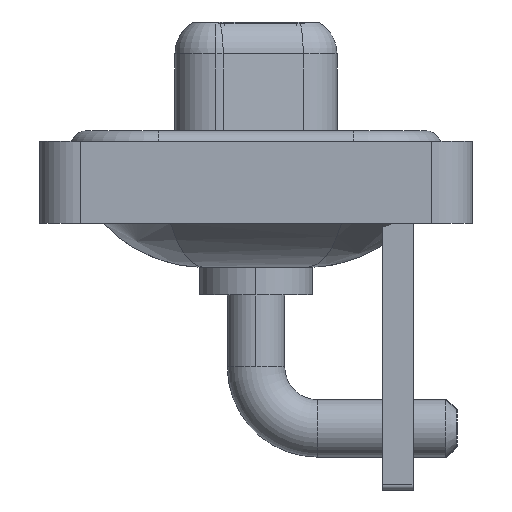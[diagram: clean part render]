
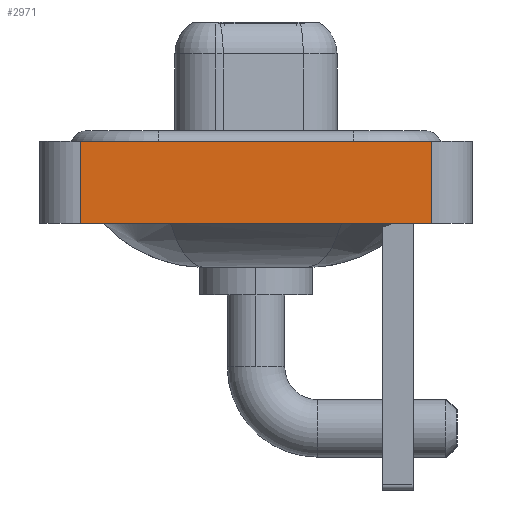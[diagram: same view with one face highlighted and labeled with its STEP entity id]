
A CAD part, left-side view. The second image highlights one B-rep face of the part: STEP entity #2971.
In plain terms, the highlighted planar face has unit normal (-1, 0, 0).
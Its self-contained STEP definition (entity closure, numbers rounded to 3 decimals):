
#791 = ORIENTED_EDGE ( 'NONE', *, *, #10012, .T. ) ;
#990 = CARTESIAN_POINT ( 'NONE',  ( -7.3, 8.55, -3.6 ) ) ;
#1152 = DIRECTION ( 'NONE',  ( 0., -1., 0. ) ) ;
#2971 = ADVANCED_FACE ( 'NONE', ( #12837 ), #17262, .T. ) ;
#3034 = CARTESIAN_POINT ( 'NONE',  ( -7.3, -8.55, -3.6 ) ) ;
#3097 = EDGE_CURVE ( 'NONE', #4671, #17338, #14737, .T. ) ;
#3956 = VECTOR ( 'NONE', #1152, 1000. ) ;
#4031 = LINE ( 'NONE', #13815, #3956 ) ;
#4326 = CARTESIAN_POINT ( 'NONE',  ( -7.3, -8.55, -3.6 ) ) ;
#4671 = VERTEX_POINT ( 'NONE', #17143 ) ;
#5493 = VERTEX_POINT ( 'NONE', #13110 ) ;
#5667 = VECTOR ( 'NONE', #5874, 1000. ) ;
#5874 = DIRECTION ( 'NONE',  ( 0., 0., 1. ) ) ;
#5879 = DIRECTION ( 'NONE',  ( 0., 0., 1. ) ) ;
#6890 = LINE ( 'NONE', #4326, #5667 ) ;
#7021 = CARTESIAN_POINT ( 'NONE',  ( -7.3, -8.55, -3.6 ) ) ;
#7369 = ORIENTED_EDGE ( 'NONE', *, *, #3097, .T. ) ;
#9213 = VECTOR ( 'NONE', #12275, 1000. ) ;
#9560 = CARTESIAN_POINT ( 'NONE',  ( -7.3, -8.55, 0.4 ) ) ;
#10012 = EDGE_CURVE ( 'NONE', #17338, #14503, #6890, .T. ) ;
#10489 = EDGE_LOOP ( 'NONE', ( #791, #13140, #17829, #7369 ) ) ;
#10796 = LINE ( 'NONE', #990, #9213 ) ;
#12275 = DIRECTION ( 'NONE',  ( 0., 0., 1. ) ) ;
#12837 = FACE_OUTER_BOUND ( 'NONE', #10489, .T. ) ;
#13016 = DIRECTION ( 'NONE',  ( -1., 0., 0. ) ) ;
#13037 = CARTESIAN_POINT ( 'NONE',  ( -7.3, -8.55, -3.6 ) ) ;
#13110 = CARTESIAN_POINT ( 'NONE',  ( -7.3, 8.55, 0.4 ) ) ;
#13140 = ORIENTED_EDGE ( 'NONE', *, *, #13371, .F. ) ;
#13371 = EDGE_CURVE ( 'NONE', #5493, #14503, #4031, .T. ) ;
#13815 = CARTESIAN_POINT ( 'NONE',  ( -7.3, -8.55, 0.4 ) ) ;
#14503 = VERTEX_POINT ( 'NONE', #9560 ) ;
#14737 = LINE ( 'NONE', #13037, #17020 ) ;
#14924 = DIRECTION ( 'NONE',  ( 0., -1., 0. ) ) ;
#15532 = AXIS2_PLACEMENT_3D ( 'NONE', #3034, #13016, #5879 ) ;
#17020 = VECTOR ( 'NONE', #14924, 1000. ) ;
#17143 = CARTESIAN_POINT ( 'NONE',  ( -7.3, 8.55, -3.6 ) ) ;
#17262 = PLANE ( 'NONE',  #15532 ) ;
#17338 = VERTEX_POINT ( 'NONE', #7021 ) ;
#17829 = ORIENTED_EDGE ( 'NONE', *, *, #18252, .F. ) ;
#18252 = EDGE_CURVE ( 'NONE', #4671, #5493, #10796, .T. ) ;
